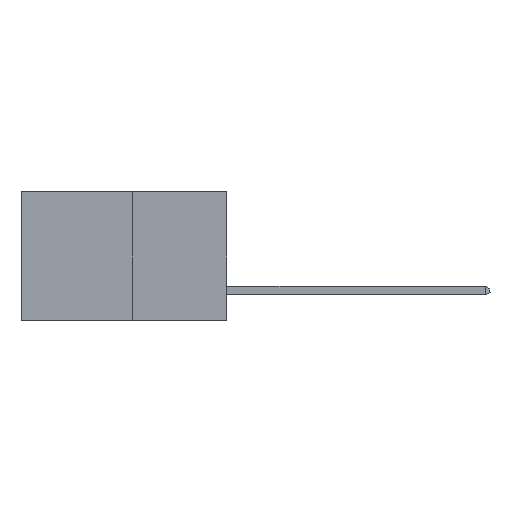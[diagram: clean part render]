
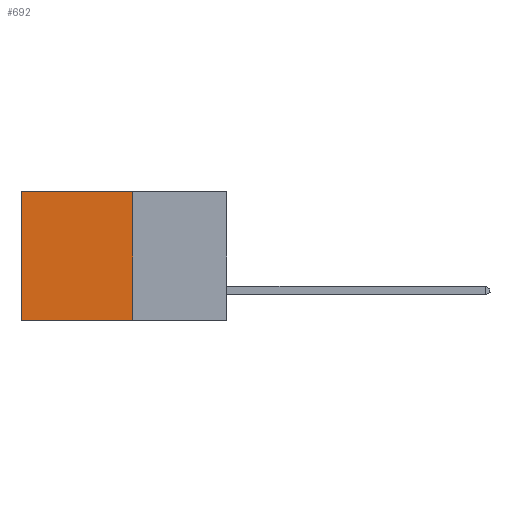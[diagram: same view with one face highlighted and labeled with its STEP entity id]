
A CAD part, left-side view. The second image highlights one B-rep face of the part: STEP entity #692.
In plain terms, the highlighted planar face has unit normal (-1, 0, 0).
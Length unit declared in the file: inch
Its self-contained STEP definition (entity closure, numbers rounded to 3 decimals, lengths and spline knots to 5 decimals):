
#368 = VERTEX_POINT ( 'NONE', #6498 ) ;
#464 = CARTESIAN_POINT ( 'NONE',  ( 0.277, 0.27, 0. ) ) ;
#692 = ADVANCED_FACE ( 'NONE', ( #2577 ), #15687, .F. ) ;
#949 = AXIS2_PLACEMENT_3D ( 'NONE', #15670, #13502, #10846 ) ;
#1024 = CARTESIAN_POINT ( 'NONE',  ( 0.277, 0.59, -0.37 ) ) ;
#2577 = FACE_OUTER_BOUND ( 'NONE', #14711, .T. ) ;
#2584 = LINE ( 'NONE', #4935, #8750 ) ;
#4234 = CARTESIAN_POINT ( 'NONE',  ( 0.277, 0.27, -0.37 ) ) ;
#4350 = DIRECTION ( 'NONE',  ( 0., 0., -1. ) ) ;
#4935 = CARTESIAN_POINT ( 'NONE',  ( 0.277, 0.27, -0.37 ) ) ;
#5269 = CARTESIAN_POINT ( 'NONE',  ( 0.277, 0.27, 0. ) ) ;
#5316 = VECTOR ( 'NONE', #14389, 39.37008 ) ;
#5336 = EDGE_CURVE ( 'NONE', #9880, #12801, #10976, .T. ) ;
#5667 = EDGE_CURVE ( 'NONE', #9880, #8698, #2584, .T. ) ;
#6498 = CARTESIAN_POINT ( 'NONE',  ( 0.277, 0.59, -0.37 ) ) ;
#6543 = DIRECTION ( 'NONE',  ( 0., 1., 0. ) ) ;
#6782 = EDGE_CURVE ( 'NONE', #12801, #368, #8914, .T. ) ;
#7285 = VECTOR ( 'NONE', #6543, 39.37008 ) ;
#7321 = ORIENTED_EDGE ( 'NONE', *, *, #6782, .T. ) ;
#8069 = ORIENTED_EDGE ( 'NONE', *, *, #5336, .T. ) ;
#8422 = CARTESIAN_POINT ( 'NONE',  ( 0.277, 0.27, -0.37 ) ) ;
#8698 = VERTEX_POINT ( 'NONE', #8422 ) ;
#8750 = VECTOR ( 'NONE', #4350, 39.37008 ) ;
#8914 = LINE ( 'NONE', #1024, #5316 ) ;
#9880 = VERTEX_POINT ( 'NONE', #464 ) ;
#10401 = CARTESIAN_POINT ( 'NONE',  ( 0.277, 0.59, 0. ) ) ;
#10479 = ORIENTED_EDGE ( 'NONE', *, *, #13427, .F. ) ;
#10846 = DIRECTION ( 'NONE',  ( 0., 0., -1. ) ) ;
#10976 = LINE ( 'NONE', #5269, #7285 ) ;
#11069 = VECTOR ( 'NONE', #15048, 39.37008 ) ;
#12801 = VERTEX_POINT ( 'NONE', #10401 ) ;
#13427 = EDGE_CURVE ( 'NONE', #8698, #368, #14224, .T. ) ;
#13502 = DIRECTION ( 'NONE',  ( 1., 0., 0. ) ) ;
#13640 = ORIENTED_EDGE ( 'NONE', *, *, #5667, .F. ) ;
#14224 = LINE ( 'NONE', #4234, #11069 ) ;
#14389 = DIRECTION ( 'NONE',  ( 0., 0., -1. ) ) ;
#14711 = EDGE_LOOP ( 'NONE', ( #7321, #10479, #13640, #8069 ) ) ;
#15048 = DIRECTION ( 'NONE',  ( 0., 1., 0. ) ) ;
#15670 = CARTESIAN_POINT ( 'NONE',  ( 0.277, 0.27, -0.37 ) ) ;
#15687 = PLANE ( 'NONE',  #949 ) ;
